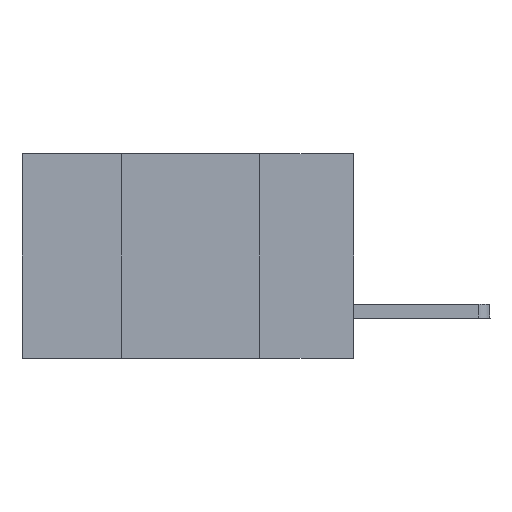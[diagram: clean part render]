
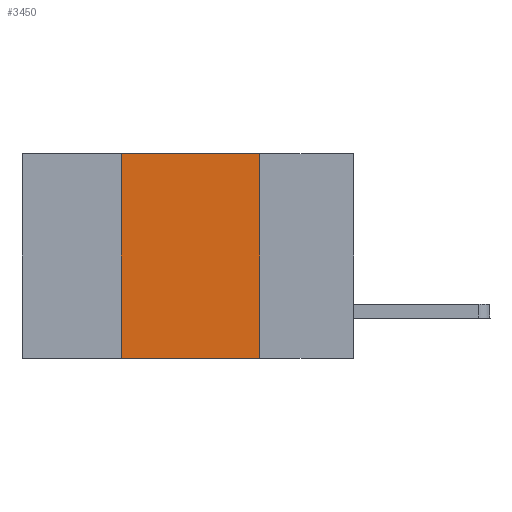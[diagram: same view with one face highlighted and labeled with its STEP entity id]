
A CAD part, left-side view. The second image highlights one B-rep face of the part: STEP entity #3450.
In plain terms, the highlighted planar face has unit normal (-1, 0, 0).
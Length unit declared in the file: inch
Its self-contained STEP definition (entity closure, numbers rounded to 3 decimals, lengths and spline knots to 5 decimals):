
#1145 = ORIENTED_EDGE ( 'NONE', *, *, #12023, .F. ) ;
#1362 = CARTESIAN_POINT ( 'NONE',  ( 0., 0.42, 0. ) ) ;
#1429 = CARTESIAN_POINT ( 'NONE',  ( 0., 0.42, -0.37 ) ) ;
#1811 = LINE ( 'NONE', #10170, #2883 ) ;
#1865 = VERTEX_POINT ( 'NONE', #8853 ) ;
#1935 = DIRECTION ( 'NONE',  ( 1., 0., 0. ) ) ;
#2013 = DIRECTION ( 'NONE',  ( 0., -1., 0. ) ) ;
#2022 = LINE ( 'NONE', #1362, #11983 ) ;
#2253 = DIRECTION ( 'NONE',  ( 0., -1., 0. ) ) ;
#2284 = DIRECTION ( 'NONE',  ( 0., 0., 1. ) ) ;
#2842 = VECTOR ( 'NONE', #2013, 39.37008 ) ;
#2883 = VECTOR ( 'NONE', #2253, 39.37008 ) ;
#3006 = CARTESIAN_POINT ( 'NONE',  ( 0., 0.17, 0. ) ) ;
#3045 = VERTEX_POINT ( 'NONE', #1429 ) ;
#3139 = AXIS2_PLACEMENT_3D ( 'NONE', #6763, #1935, #9584 ) ;
#3447 = VECTOR ( 'NONE', #3873, 39.37008 ) ;
#3450 = ADVANCED_FACE ( 'NONE', ( #8787 ), #3990, .F. ) ;
#3873 = DIRECTION ( 'NONE',  ( 0., 0., -1. ) ) ;
#3990 = PLANE ( 'NONE',  #3139 ) ;
#4121 = VERTEX_POINT ( 'NONE', #7407 ) ;
#4355 = LINE ( 'NONE', #7894, #2842 ) ;
#4489 = EDGE_CURVE ( 'NONE', #3045, #1865, #4355, .T. ) ;
#4796 = ORIENTED_EDGE ( 'NONE', *, *, #10130, .F. ) ;
#5925 = ORIENTED_EDGE ( 'NONE', *, *, #7228, .F. ) ;
#6763 = CARTESIAN_POINT ( 'NONE',  ( 0., 0.6, 0. ) ) ;
#7228 = EDGE_CURVE ( 'NONE', #4121, #1865, #12187, .T. ) ;
#7377 = EDGE_LOOP ( 'NONE', ( #5925, #1145, #4796, #12228 ) ) ;
#7407 = CARTESIAN_POINT ( 'NONE',  ( 0., 0.17, 0. ) ) ;
#7894 = CARTESIAN_POINT ( 'NONE',  ( 0., 0.6, -0.37 ) ) ;
#8787 = FACE_OUTER_BOUND ( 'NONE', #7377, .T. ) ;
#8853 = CARTESIAN_POINT ( 'NONE',  ( 0., 0.17, -0.37 ) ) ;
#9545 = VERTEX_POINT ( 'NONE', #10849 ) ;
#9584 = DIRECTION ( 'NONE',  ( 0., 0., -1. ) ) ;
#10130 = EDGE_CURVE ( 'NONE', #3045, #9545, #2022, .T. ) ;
#10170 = CARTESIAN_POINT ( 'NONE',  ( 0., 0.6, 0. ) ) ;
#10849 = CARTESIAN_POINT ( 'NONE',  ( 0., 0.42, 0. ) ) ;
#11983 = VECTOR ( 'NONE', #2284, 39.37008 ) ;
#12023 = EDGE_CURVE ( 'NONE', #9545, #4121, #1811, .T. ) ;
#12187 = LINE ( 'NONE', #3006, #3447 ) ;
#12228 = ORIENTED_EDGE ( 'NONE', *, *, #4489, .T. ) ;
